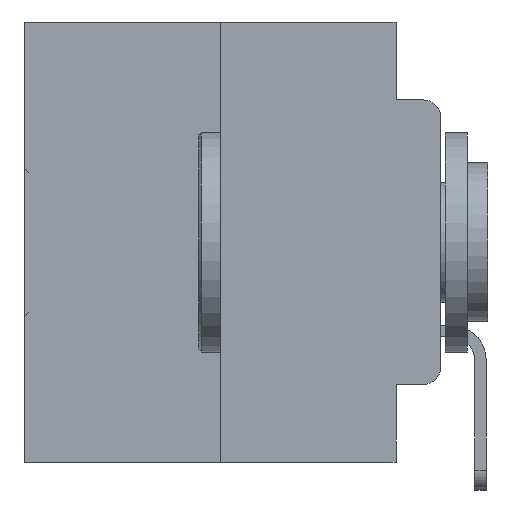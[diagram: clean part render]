
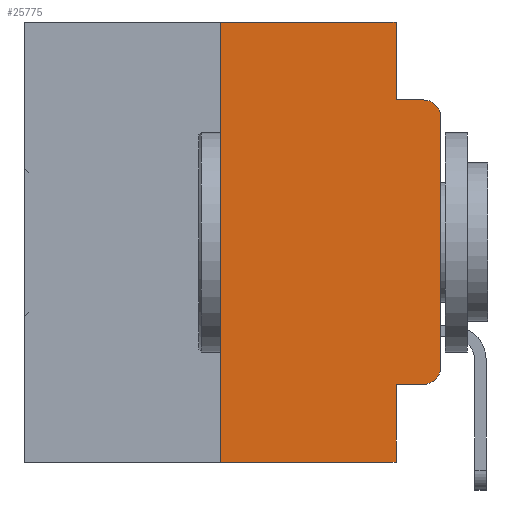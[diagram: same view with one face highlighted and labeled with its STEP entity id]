
A CAD part, left-side view. The second image highlights one B-rep face of the part: STEP entity #25775.
In plain terms, the highlighted planar face has unit normal (-1, 0, 0).
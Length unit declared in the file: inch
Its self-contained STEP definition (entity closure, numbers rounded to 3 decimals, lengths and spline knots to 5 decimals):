
#221 = VECTOR ( 'NONE', #2209, 39.37008 ) ;
#248 = DIRECTION ( 'NONE',  ( -1., 0., 0. ) ) ;
#435 = LINE ( 'NONE', #14942, #24754 ) ;
#466 = CARTESIAN_POINT ( 'NONE',  ( 0., 0.051, -0.5 ) ) ;
#877 = VERTEX_POINT ( 'NONE', #24817 ) ;
#1017 = VERTEX_POINT ( 'NONE', #11077 ) ;
#1303 = EDGE_CURVE ( 'NONE', #13679, #15528, #5016, .T. ) ;
#1822 = VECTOR ( 'NONE', #31590, 39.37008 ) ;
#2086 = CARTESIAN_POINT ( 'NONE',  ( 0., 0.051, -0.4115 ) ) ;
#2145 = VERTEX_POINT ( 'NONE', #13213 ) ;
#2209 = DIRECTION ( 'NONE',  ( 0., 0., 1. ) ) ;
#2753 = DIRECTION ( 'NONE',  ( 0., 0., -1. ) ) ;
#2861 = ORIENTED_EDGE ( 'NONE', *, *, #21771, .F. ) ;
#2968 = CARTESIAN_POINT ( 'NONE',  ( 0., 0.051, -0.0885 ) ) ;
#3415 = CARTESIAN_POINT ( 'NONE',  ( 0., 0.02, -0.0885 ) ) ;
#3841 = CARTESIAN_POINT ( 'NONE',  ( 0., 0.473, -0.5 ) ) ;
#4402 = CARTESIAN_POINT ( 'NONE',  ( 0., 0.25, -0.5 ) ) ;
#4648 = VECTOR ( 'NONE', #16699, 39.37008 ) ;
#5016 = LINE ( 'NONE', #22315, #30157 ) ;
#5050 = CARTESIAN_POINT ( 'NONE',  ( 0., 0.051, 0. ) ) ;
#5180 = CIRCLE ( 'NONE', #26623, 0.02 ) ;
#5504 = DIRECTION ( 'NONE',  ( 1., 0., 0. ) ) ;
#5831 = VECTOR ( 'NONE', #28729, 39.37008 ) ;
#6782 = EDGE_CURVE ( 'NONE', #28528, #12155, #10539, .T. ) ;
#6888 = CARTESIAN_POINT ( 'NONE',  ( 0., 0.051, -0.4115 ) ) ;
#7229 = ORIENTED_EDGE ( 'NONE', *, *, #6782, .F. ) ;
#7528 = CARTESIAN_POINT ( 'NONE',  ( 0., 0., 0. ) ) ;
#7859 = CARTESIAN_POINT ( 'NONE',  ( 0., 0.25, 0. ) ) ;
#8076 = CARTESIAN_POINT ( 'NONE',  ( 0., 0.473, 0. ) ) ;
#8444 = VECTOR ( 'NONE', #30879, 39.37008 ) ;
#8819 = ORIENTED_EDGE ( 'NONE', *, *, #28401, .T. ) ;
#9171 = VECTOR ( 'NONE', #9988, 39.37008 ) ;
#9322 = FACE_OUTER_BOUND ( 'NONE', #11534, .T. ) ;
#9988 = DIRECTION ( 'NONE',  ( 0., 0., -1. ) ) ;
#10539 = LINE ( 'NONE', #15133, #1822 ) ;
#11077 = CARTESIAN_POINT ( 'NONE',  ( 0., 0.02, -0.4115 ) ) ;
#11081 = EDGE_CURVE ( 'NONE', #1017, #2145, #5180, .T. ) ;
#11181 = VERTEX_POINT ( 'NONE', #466 ) ;
#11534 = EDGE_LOOP ( 'NONE', ( #8819, #15548, #22161, #29884, #7229, #15606, #25528, #2861, #22434, #30532 ) ) ;
#12155 = VERTEX_POINT ( 'NONE', #5050 ) ;
#12489 = EDGE_CURVE ( 'NONE', #26730, #11181, #15183, .T. ) ;
#12642 = EDGE_CURVE ( 'NONE', #26730, #28528, #435, .T. ) ;
#12761 = LINE ( 'NONE', #6888, #5831 ) ;
#13213 = CARTESIAN_POINT ( 'NONE',  ( 0., 0., -0.3915 ) ) ;
#13269 = EDGE_CURVE ( 'NONE', #12155, #13679, #30570, .T. ) ;
#13679 = VERTEX_POINT ( 'NONE', #2968 ) ;
#14286 = CARTESIAN_POINT ( 'NONE',  ( 0., 0.051, 0. ) ) ;
#14942 = CARTESIAN_POINT ( 'NONE',  ( 0., 0.25, 0. ) ) ;
#15133 = CARTESIAN_POINT ( 'NONE',  ( 0., 0.473, 0. ) ) ;
#15183 = LINE ( 'NONE', #3841, #8444 ) ;
#15215 = DIRECTION ( 'NONE',  ( 0., -1., 0. ) ) ;
#15528 = VERTEX_POINT ( 'NONE', #3415 ) ;
#15548 = ORIENTED_EDGE ( 'NONE', *, *, #22782, .T. ) ;
#15606 = ORIENTED_EDGE ( 'NONE', *, *, #12642, .F. ) ;
#15719 = PLANE ( 'NONE',  #18633 ) ;
#15875 = CARTESIAN_POINT ( 'NONE',  ( 0., 0.02, -0.1085 ) ) ;
#16699 = DIRECTION ( 'NONE',  ( 0., 0., -1. ) ) ;
#18052 = DIRECTION ( 'NONE',  ( -1., 0., 0. ) ) ;
#18253 = DIRECTION ( 'NONE',  ( 0., 0., -1. ) ) ;
#18633 = AXIS2_PLACEMENT_3D ( 'NONE', #8076, #5504, #22792 ) ;
#20513 = LINE ( 'NONE', #7528, #221 ) ;
#20583 = CIRCLE ( 'NONE', #21702, 0.02 ) ;
#21702 = AXIS2_PLACEMENT_3D ( 'NONE', #15875, #248, #18253 ) ;
#21771 = EDGE_CURVE ( 'NONE', #24637, #11181, #22108, .T. ) ;
#22108 = LINE ( 'NONE', #26818, #9171 ) ;
#22161 = ORIENTED_EDGE ( 'NONE', *, *, #1303, .F. ) ;
#22315 = CARTESIAN_POINT ( 'NONE',  ( 0., 0.051, -0.0885 ) ) ;
#22370 = EDGE_CURVE ( 'NONE', #24637, #1017, #12761, .T. ) ;
#22434 = ORIENTED_EDGE ( 'NONE', *, *, #22370, .T. ) ;
#22782 = EDGE_CURVE ( 'NONE', #877, #15528, #20583, .T. ) ;
#22792 = DIRECTION ( 'NONE',  ( 0., 0., -1. ) ) ;
#24637 = VERTEX_POINT ( 'NONE', #2086 ) ;
#24754 = VECTOR ( 'NONE', #26672, 39.37008 ) ;
#24817 = CARTESIAN_POINT ( 'NONE',  ( 0., 0., -0.1085 ) ) ;
#25528 = ORIENTED_EDGE ( 'NONE', *, *, #12489, .T. ) ;
#25775 = ADVANCED_FACE ( 'NONE', ( #9322 ), #15719, .F. ) ;
#26623 = AXIS2_PLACEMENT_3D ( 'NONE', #32073, #18052, #2753 ) ;
#26672 = DIRECTION ( 'NONE',  ( 0., 0., 1. ) ) ;
#26730 = VERTEX_POINT ( 'NONE', #4402 ) ;
#26818 = CARTESIAN_POINT ( 'NONE',  ( 0., 0.051, 0. ) ) ;
#28401 = EDGE_CURVE ( 'NONE', #2145, #877, #20513, .T. ) ;
#28528 = VERTEX_POINT ( 'NONE', #7859 ) ;
#28729 = DIRECTION ( 'NONE',  ( 0., -1., 0. ) ) ;
#29884 = ORIENTED_EDGE ( 'NONE', *, *, #13269, .F. ) ;
#30157 = VECTOR ( 'NONE', #15215, 39.37008 ) ;
#30532 = ORIENTED_EDGE ( 'NONE', *, *, #11081, .T. ) ;
#30570 = LINE ( 'NONE', #14286, #4648 ) ;
#30879 = DIRECTION ( 'NONE',  ( 0., -1., 0. ) ) ;
#31590 = DIRECTION ( 'NONE',  ( 0., -1., 0. ) ) ;
#32073 = CARTESIAN_POINT ( 'NONE',  ( 0., 0.02, -0.3915 ) ) ;
